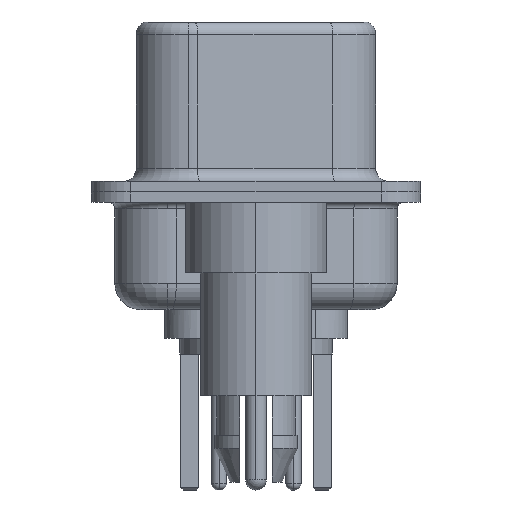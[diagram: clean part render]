
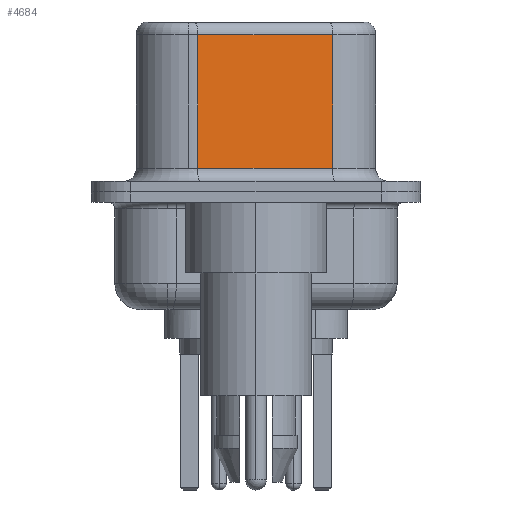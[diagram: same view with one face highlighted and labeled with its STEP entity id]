
A CAD part, left-side view. The second image highlights one B-rep face of the part: STEP entity #4684.
In plain terms, the highlighted planar face has unit normal (-0.985, -0.174, 0).
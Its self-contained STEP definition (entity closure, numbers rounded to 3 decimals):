
#398 = VERTEX_POINT ( 'NONE', #4036 ) ;
#665 = EDGE_CURVE ( 'NONE', #8295, #398, #20242, .T. ) ;
#3455 = DIRECTION ( 'NONE',  ( 0.985, 0.174, 0. ) ) ;
#4036 = CARTESIAN_POINT ( 'NONE',  ( 4.585, -2.927, 0.9 ) ) ;
#4635 = CARTESIAN_POINT ( 'NONE',  ( 4.585, -2.927, 6.52 ) ) ;
#4678 = PLANE ( 'NONE',  #16669 ) ;
#4684 = ADVANCED_FACE ( 'NONE', ( #9598 ), #4678, .F. ) ;
#4927 = VERTEX_POINT ( 'NONE', #9052 ) ;
#5638 = VERTEX_POINT ( 'NONE', #20666 ) ;
#5825 = CARTESIAN_POINT ( 'NONE',  ( 3.675, 2.233, 6.52 ) ) ;
#6348 = DIRECTION ( 'NONE',  ( 0., 0., -1. ) ) ;
#7023 = ORIENTED_EDGE ( 'NONE', *, *, #665, .T. ) ;
#8177 = DIRECTION ( 'NONE',  ( -0.174, 0.985, 0. ) ) ;
#8295 = VERTEX_POINT ( 'NONE', #13266 ) ;
#9052 = CARTESIAN_POINT ( 'NONE',  ( 4.585, -2.927, 6.02 ) ) ;
#9427 = LINE ( 'NONE', #5825, #17110 ) ;
#9598 = FACE_OUTER_BOUND ( 'NONE', #13943, .T. ) ;
#13266 = CARTESIAN_POINT ( 'NONE',  ( 3.675, 2.233, 0.9 ) ) ;
#13420 = EDGE_CURVE ( 'NONE', #5638, #8295, #9427, .T. ) ;
#13544 = VECTOR ( 'NONE', #6348, 1000. ) ;
#13634 = VECTOR ( 'NONE', #14260, 1000. ) ;
#13943 = EDGE_LOOP ( 'NONE', ( #20595, #16522, #20793, #7023 ) ) ;
#14040 = CARTESIAN_POINT ( 'NONE',  ( 4.585, -2.927, 6.52 ) ) ;
#14260 = DIRECTION ( 'NONE',  ( -0.174, 0.985, 0. ) ) ;
#14570 = DIRECTION ( 'NONE',  ( 0., 0., -1. ) ) ;
#15241 = VECTOR ( 'NONE', #22392, 1000. ) ;
#16522 = ORIENTED_EDGE ( 'NONE', *, *, #19878, .T. ) ;
#16669 = AXIS2_PLACEMENT_3D ( 'NONE', #14040, #3455, #8177 ) ;
#17110 = VECTOR ( 'NONE', #14570, 1000. ) ;
#18244 = LINE ( 'NONE', #4635, #13544 ) ;
#18785 = CARTESIAN_POINT ( 'NONE',  ( 4.585, -2.927, 0.9 ) ) ;
#19878 = EDGE_CURVE ( 'NONE', #4927, #5638, #21997, .T. ) ;
#20242 = LINE ( 'NONE', #18785, #15241 ) ;
#20595 = ORIENTED_EDGE ( 'NONE', *, *, #22217, .F. ) ;
#20666 = CARTESIAN_POINT ( 'NONE',  ( 3.675, 2.233, 6.02 ) ) ;
#20793 = ORIENTED_EDGE ( 'NONE', *, *, #13420, .T. ) ;
#21168 = CARTESIAN_POINT ( 'NONE',  ( 4.585, -2.927, 6.02 ) ) ;
#21997 = LINE ( 'NONE', #21168, #13634 ) ;
#22217 = EDGE_CURVE ( 'NONE', #4927, #398, #18244, .T. ) ;
#22392 = DIRECTION ( 'NONE',  ( 0.174, -0.985, 0. ) ) ;
